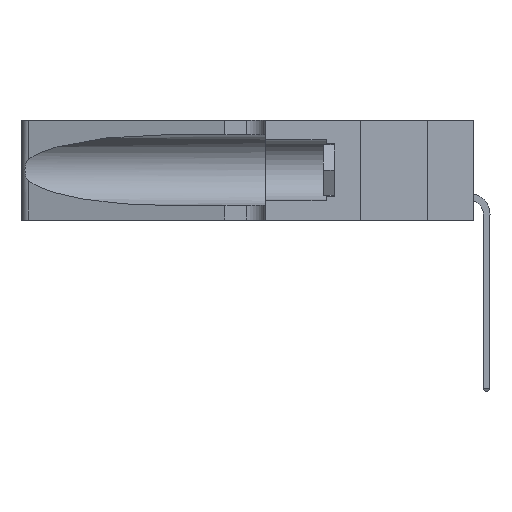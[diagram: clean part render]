
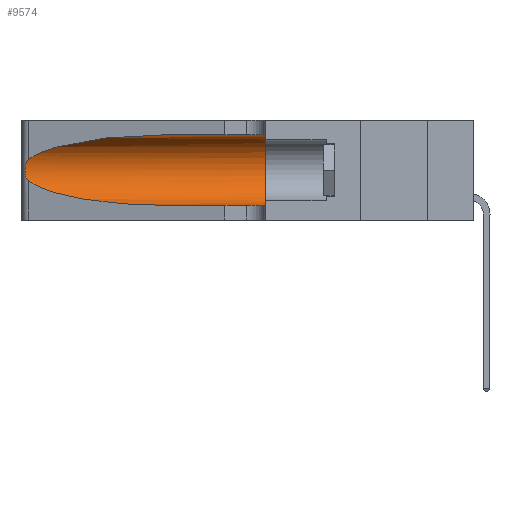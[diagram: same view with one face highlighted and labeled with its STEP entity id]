
A CAD part, left-side view. The second image highlights one B-rep face of the part: STEP entity #9574.
In plain terms, the highlighted cylindrical face has radius 3.308 mm (diameter 6.617 mm), a partial arc.
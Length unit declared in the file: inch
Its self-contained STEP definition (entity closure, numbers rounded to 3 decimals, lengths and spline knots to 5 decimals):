
#1250 = DIRECTION ( 'NONE',  ( 0., -1., 0. ) ) ;
#1338 = CARTESIAN_POINT ( 'NONE',  ( 0.25787, 1.23484, 0.2124 ) ) ;
#1608 = CARTESIAN_POINT ( 'NONE',  ( 0.1305, 0.35, 0.05475 ) ) ;
#2127 = B_SPLINE_CURVE_WITH_KNOTS ( 'NONE', 3,
 ( #27154, #14388, #12213, #1338, #9846, #5541, #22926, #27249, #14286, #3219, #24698, #16355, #22831, #5373 ),
 .UNSPECIFIED., .F., .F.,
 ( 4, 2, 2, 2, 2, 2, 4 ),
 ( 0., 0.00027, 0.00053, 0.00107, 0.0016, 0.00187, 0.00214 ),
 .UNSPECIFIED. ) ;
#2182 = AXIS2_PLACEMENT_3D ( 'NONE', #26025, #8825, #12966 ) ;
#2701 = FACE_OUTER_BOUND ( 'NONE', #19531, .T. ) ;
#2831 = EDGE_CURVE ( 'NONE', #13240, #3695, #5664, .T. ) ;
#2859 = CARTESIAN_POINT ( 'NONE',  ( 0.18966, 0.96281, 0.05475 ) ) ;
#3077 = DIRECTION ( 'NONE',  ( 0., -1., 0. ) ) ;
#3219 = CARTESIAN_POINT ( 'NONE',  ( 0.25856, 1.23593, 0.16098 ) ) ;
#3695 = VERTEX_POINT ( 'NONE', #1608 ) ;
#5373 = CARTESIAN_POINT ( 'NONE',  ( 0.25487, 1.22718, 0.14631 ) ) ;
#5541 = CARTESIAN_POINT ( 'NONE',  ( 0.26018, 1.23835, 0.19895 ) ) ;
#5609 = VERTEX_POINT ( 'NONE', #15140 ) ;
#5664 = CIRCLE ( 'NONE', #13052, 0.13025 ) ;
#6333 = LINE ( 'NONE', #7272, #12737 ) ;
#6393 =( BOUNDED_CURVE ( )  B_SPLINE_CURVE ( 3, ( #26465, #7185, #15844, #20175 ),
 .UNSPECIFIED., .F., .T. ) 
 B_SPLINE_CURVE_WITH_KNOTS ( ( 4, 4 ),
 ( 1.5708, 2.84003 ),
 .UNSPECIFIED. ) 
 CURVE ( )  GEOMETRIC_REPRESENTATION_ITEM ( )  RATIONAL_B_SPLINE_CURVE ( ( 1., 0.87, 0.87, 1. ) ) 
 REPRESENTATION_ITEM ( '' )  );
#7185 = CARTESIAN_POINT ( 'NONE',  ( 0.18966, 0.96281, 0.31525 ) ) ;
#7272 = CARTESIAN_POINT ( 'NONE',  ( 0.1305, 1.61858, 0.31525 ) ) ;
#8796 = CARTESIAN_POINT ( 'NONE',  ( 0.1305, 0.35, 0.31525 ) ) ;
#8825 = DIRECTION ( 'NONE',  ( 0., -1., 0. ) ) ;
#9574 = ADVANCED_FACE ( 'NONE', ( #2701 ), #14802, .F. ) ;
#9846 = CARTESIAN_POINT ( 'NONE',  ( 0.25854, 1.2359, 0.20912 ) ) ;
#10135 = EDGE_CURVE ( 'NONE', #16364, #13240, #6333, .T. ) ;
#10632 = EDGE_CURVE ( 'NONE', #16364, #5609, #6393, .T. ) ;
#12213 = CARTESIAN_POINT ( 'NONE',  ( 0.25639, 1.23184, 0.21858 ) ) ;
#12737 = VECTOR ( 'NONE', #3077, 39.37008 ) ;
#12966 = DIRECTION ( 'NONE',  ( 0., 0., -1. ) ) ;
#13052 = AXIS2_PLACEMENT_3D ( 'NONE', #27479, #16592, #27391 ) ;
#13240 = VERTEX_POINT ( 'NONE', #8796 ) ;
#13821 = EDGE_CURVE ( 'NONE', #5609, #27106, #2127, .T. ) ;
#13882 = EDGE_CURVE ( 'NONE', #23948, #3695, #22683, .T. ) ;
#14286 = CARTESIAN_POINT ( 'NONE',  ( 0.26017, 1.23833, 0.17102 ) ) ;
#14388 = CARTESIAN_POINT ( 'NONE',  ( 0.25555, 1.22994, 0.2215 ) ) ;
#14391 = CARTESIAN_POINT ( 'NONE',  ( 0.1305, 0.72297, 0.31525 ) ) ;
#14663 = ORIENTED_EDGE ( 'NONE', *, *, #13821, .T. ) ;
#14802 = CYLINDRICAL_SURFACE ( 'NONE', #2182, 0.13025 ) ;
#15062 =( BOUNDED_CURVE ( )  B_SPLINE_CURVE ( 3, ( #23980, #26255, #2859, #17893 ),
 .UNSPECIFIED., .F., .F. ) 
 B_SPLINE_CURVE_WITH_KNOTS ( ( 4, 4 ),
 ( 3.44316, 4.71239 ),
 .UNSPECIFIED. ) 
 CURVE ( )  GEOMETRIC_REPRESENTATION_ITEM ( )  RATIONAL_B_SPLINE_CURVE ( ( 1., 0.87, 0.87, 1. ) ) 
 REPRESENTATION_ITEM ( '' )  );
#15140 = CARTESIAN_POINT ( 'NONE',  ( 0.25487, 1.22718, 0.22369 ) ) ;
#15844 = CARTESIAN_POINT ( 'NONE',  ( 0.2373, 1.15595, 0.28018 ) ) ;
#16355 = CARTESIAN_POINT ( 'NONE',  ( 0.25639, 1.23186, 0.15144 ) ) ;
#16364 = VERTEX_POINT ( 'NONE', #14391 ) ;
#16592 = DIRECTION ( 'NONE',  ( 0., 1., 0. ) ) ;
#17893 = CARTESIAN_POINT ( 'NONE',  ( 0.1305, 0.72297, 0.05475 ) ) ;
#18091 = ORIENTED_EDGE ( 'NONE', *, *, #21297, .T. ) ;
#18983 = VECTOR ( 'NONE', #1250, 39.37008 ) ;
#19531 = EDGE_LOOP ( 'NONE', ( #26782, #14663, #18091, #20907, #27613, #20557 ) ) ;
#20175 = CARTESIAN_POINT ( 'NONE',  ( 0.25487, 1.22718, 0.22369 ) ) ;
#20557 = ORIENTED_EDGE ( 'NONE', *, *, #10135, .F. ) ;
#20907 = ORIENTED_EDGE ( 'NONE', *, *, #13882, .T. ) ;
#21297 = EDGE_CURVE ( 'NONE', #27106, #23948, #15062, .T. ) ;
#22567 = CARTESIAN_POINT ( 'NONE',  ( 0.1305, 1.61858, 0.05475 ) ) ;
#22683 = LINE ( 'NONE', #22567, #18983 ) ;
#22831 = CARTESIAN_POINT ( 'NONE',  ( 0.25555, 1.22993, 0.14849 ) ) ;
#22926 = CARTESIAN_POINT ( 'NONE',  ( 0.26075, 1.23896, 0.19203 ) ) ;
#23689 = CARTESIAN_POINT ( 'NONE',  ( 0.1305, 0.72297, 0.05475 ) ) ;
#23948 = VERTEX_POINT ( 'NONE', #23689 ) ;
#23980 = CARTESIAN_POINT ( 'NONE',  ( 0.25487, 1.22718, 0.14631 ) ) ;
#24698 = CARTESIAN_POINT ( 'NONE',  ( 0.25789, 1.23486, 0.15765 ) ) ;
#25650 = CARTESIAN_POINT ( 'NONE',  ( 0.25487, 1.22718, 0.14631 ) ) ;
#26025 = CARTESIAN_POINT ( 'NONE',  ( 0.1305, 1.61858, 0.185 ) ) ;
#26255 = CARTESIAN_POINT ( 'NONE',  ( 0.2373, 1.15595, 0.08982 ) ) ;
#26465 = CARTESIAN_POINT ( 'NONE',  ( 0.1305, 0.72297, 0.31525 ) ) ;
#26782 = ORIENTED_EDGE ( 'NONE', *, *, #10632, .T. ) ;
#27106 = VERTEX_POINT ( 'NONE', #25650 ) ;
#27154 = CARTESIAN_POINT ( 'NONE',  ( 0.25487, 1.22718, 0.22369 ) ) ;
#27249 = CARTESIAN_POINT ( 'NONE',  ( 0.26075, 1.23896, 0.178 ) ) ;
#27391 = DIRECTION ( 'NONE',  ( 0., 0., 1. ) ) ;
#27479 = CARTESIAN_POINT ( 'NONE',  ( 0.1305, 0.35, 0.185 ) ) ;
#27613 = ORIENTED_EDGE ( 'NONE', *, *, #2831, .F. ) ;
